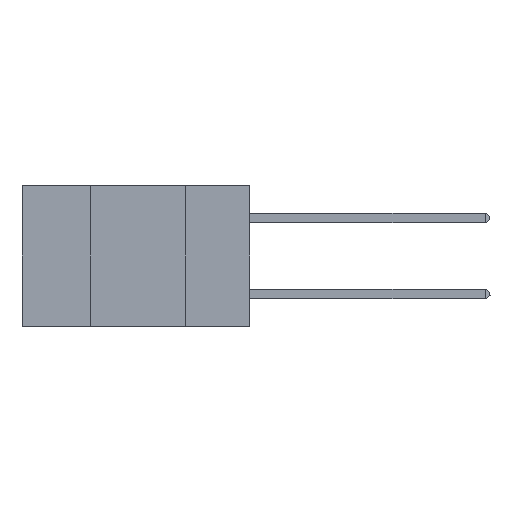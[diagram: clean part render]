
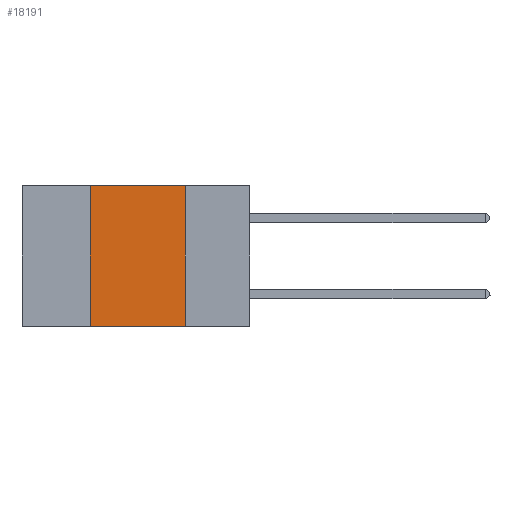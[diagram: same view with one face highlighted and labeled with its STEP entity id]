
A CAD part, left-side view. The second image highlights one B-rep face of the part: STEP entity #18191.
In plain terms, the highlighted planar face has unit normal (-1, 0, 0).
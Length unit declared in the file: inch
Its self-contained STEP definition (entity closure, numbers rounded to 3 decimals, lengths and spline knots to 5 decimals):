
#901 = DIRECTION ( 'NONE',  ( 0., 0., 1. ) ) ;
#8149 = CARTESIAN_POINT ( 'NONE',  ( 0., 0.6, -0.37 ) ) ;
#8398 = VERTEX_POINT ( 'NONE', #17416 ) ;
#9240 = DIRECTION ( 'NONE',  ( 0., 0., -1. ) ) ;
#10161 = CARTESIAN_POINT ( 'NONE',  ( 0., 0.42, -0.37 ) ) ;
#12605 = VECTOR ( 'NONE', #901, 39.37008 ) ;
#13704 = DIRECTION ( 'NONE',  ( 1., 0., 0. ) ) ;
#15021 = ORIENTED_EDGE ( 'NONE', *, *, #22899, .F. ) ;
#15337 = CARTESIAN_POINT ( 'NONE',  ( 0., 0.17, -0.37 ) ) ;
#15911 = LINE ( 'NONE', #38817, #38483 ) ;
#16228 = EDGE_CURVE ( 'NONE', #31378, #26362, #15911, .T. ) ;
#16542 = AXIS2_PLACEMENT_3D ( 'NONE', #23415, #13704, #30763 ) ;
#17301 = LINE ( 'NONE', #30476, #12605 ) ;
#17416 = CARTESIAN_POINT ( 'NONE',  ( 0., 0.42, 0. ) ) ;
#17938 = EDGE_CURVE ( 'NONE', #8398, #31378, #35327, .T. ) ;
#18191 = ADVANCED_FACE ( 'NONE', ( #30118 ), #36817, .F. ) ;
#22899 = EDGE_CURVE ( 'NONE', #39376, #8398, #17301, .T. ) ;
#23415 = CARTESIAN_POINT ( 'NONE',  ( 0., 0.6, 0. ) ) ;
#24979 = CARTESIAN_POINT ( 'NONE',  ( 0., 0.6, 0. ) ) ;
#26362 = VERTEX_POINT ( 'NONE', #15337 ) ;
#27734 = ORIENTED_EDGE ( 'NONE', *, *, #16228, .F. ) ;
#28015 = DIRECTION ( 'NONE',  ( 0., -1., 0. ) ) ;
#28381 = EDGE_CURVE ( 'NONE', #39376, #26362, #41401, .T. ) ;
#30118 = FACE_OUTER_BOUND ( 'NONE', #38523, .T. ) ;
#30476 = CARTESIAN_POINT ( 'NONE',  ( 0., 0.42, 0. ) ) ;
#30763 = DIRECTION ( 'NONE',  ( 0., 0., -1. ) ) ;
#31378 = VERTEX_POINT ( 'NONE', #40137 ) ;
#34488 = DIRECTION ( 'NONE',  ( 0., -1., 0. ) ) ;
#35327 = LINE ( 'NONE', #24979, #35816 ) ;
#35816 = VECTOR ( 'NONE', #28015, 39.37008 ) ;
#36673 = ORIENTED_EDGE ( 'NONE', *, *, #28381, .T. ) ;
#36817 = PLANE ( 'NONE',  #16542 ) ;
#37630 = VECTOR ( 'NONE', #34488, 39.37008 ) ;
#38483 = VECTOR ( 'NONE', #9240, 39.37008 ) ;
#38523 = EDGE_LOOP ( 'NONE', ( #27734, #39031, #15021, #36673 ) ) ;
#38817 = CARTESIAN_POINT ( 'NONE',  ( 0., 0.17, 0. ) ) ;
#39031 = ORIENTED_EDGE ( 'NONE', *, *, #17938, .F. ) ;
#39376 = VERTEX_POINT ( 'NONE', #10161 ) ;
#40137 = CARTESIAN_POINT ( 'NONE',  ( 0., 0.17, 0. ) ) ;
#41401 = LINE ( 'NONE', #8149, #37630 ) ;
